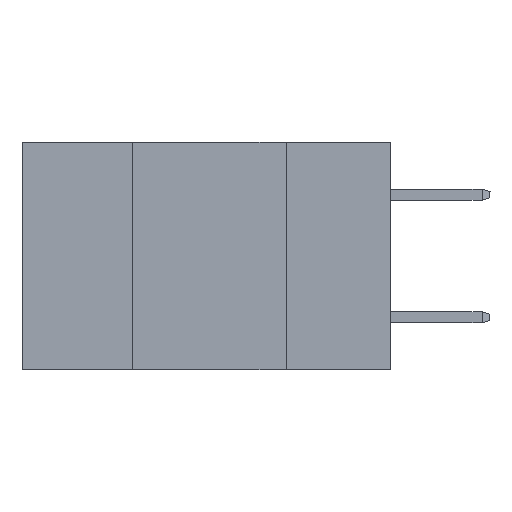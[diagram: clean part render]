
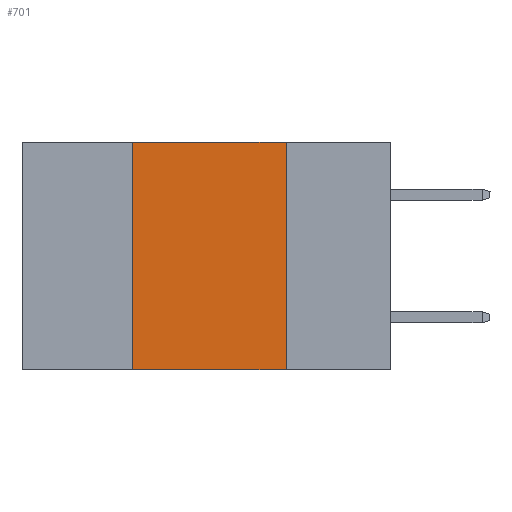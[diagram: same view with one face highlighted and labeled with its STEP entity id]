
A CAD part, left-side view. The second image highlights one B-rep face of the part: STEP entity #701.
In plain terms, the highlighted planar face has unit normal (-1, 0, 0).
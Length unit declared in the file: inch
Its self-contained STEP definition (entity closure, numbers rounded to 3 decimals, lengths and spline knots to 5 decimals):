
#64 = LINE ( 'NONE', #5505, #826 ) ;
#701 = ADVANCED_FACE ( 'NONE', ( #5177 ), #5519, .F. ) ;
#825 = VECTOR ( 'NONE', #9366, 39.37008 ) ;
#826 = VECTOR ( 'NONE', #6324, 39.37008 ) ;
#1001 = LINE ( 'NONE', #8218, #5289 ) ;
#1124 = CARTESIAN_POINT ( 'NONE',  ( 0., 0.6, -0.37 ) ) ;
#1173 = ORIENTED_EDGE ( 'NONE', *, *, #5974, .F. ) ;
#1930 = VERTEX_POINT ( 'NONE', #3570 ) ;
#2139 = CARTESIAN_POINT ( 'NONE',  ( 0., 0.6, 0. ) ) ;
#2370 = CARTESIAN_POINT ( 'NONE',  ( 0., 0.6, 0. ) ) ;
#2545 = EDGE_CURVE ( 'NONE', #3255, #5693, #4524, .T. ) ;
#2856 = EDGE_CURVE ( 'NONE', #4542, #1930, #6290, .T. ) ;
#3011 = DIRECTION ( 'NONE',  ( 0., 0., -1. ) ) ;
#3255 = VERTEX_POINT ( 'NONE', #3882 ) ;
#3570 = CARTESIAN_POINT ( 'NONE',  ( 0., 0.17, 0. ) ) ;
#3882 = CARTESIAN_POINT ( 'NONE',  ( 0., 0.42, -0.37 ) ) ;
#4016 = DIRECTION ( 'NONE',  ( 0., -1., 0. ) ) ;
#4229 = ORIENTED_EDGE ( 'NONE', *, *, #7772, .F. ) ;
#4290 = CARTESIAN_POINT ( 'NONE',  ( 0., 0.17, -0.37 ) ) ;
#4524 = LINE ( 'NONE', #1124, #7410 ) ;
#4542 = VERTEX_POINT ( 'NONE', #6496 ) ;
#5177 = FACE_OUTER_BOUND ( 'NONE', #7313, .T. ) ;
#5289 = VECTOR ( 'NONE', #9020, 39.37008 ) ;
#5505 = CARTESIAN_POINT ( 'NONE',  ( 0., 0.17, 0. ) ) ;
#5519 = PLANE ( 'NONE',  #9348 ) ;
#5693 = VERTEX_POINT ( 'NONE', #4290 ) ;
#5974 = EDGE_CURVE ( 'NONE', #3255, #4542, #1001, .T. ) ;
#6290 = LINE ( 'NONE', #2139, #825 ) ;
#6324 = DIRECTION ( 'NONE',  ( 0., 0., -1. ) ) ;
#6496 = CARTESIAN_POINT ( 'NONE',  ( 0., 0.42, 0. ) ) ;
#7313 = EDGE_LOOP ( 'NONE', ( #4229, #9362, #1173, #8686 ) ) ;
#7410 = VECTOR ( 'NONE', #4016, 39.37008 ) ;
#7772 = EDGE_CURVE ( 'NONE', #1930, #5693, #64, .T. ) ;
#7963 = DIRECTION ( 'NONE',  ( 1., 0., 0. ) ) ;
#8218 = CARTESIAN_POINT ( 'NONE',  ( 0., 0.42, 0. ) ) ;
#8686 = ORIENTED_EDGE ( 'NONE', *, *, #2545, .T. ) ;
#9020 = DIRECTION ( 'NONE',  ( 0., 0., 1. ) ) ;
#9348 = AXIS2_PLACEMENT_3D ( 'NONE', #2370, #7963, #3011 ) ;
#9362 = ORIENTED_EDGE ( 'NONE', *, *, #2856, .F. ) ;
#9366 = DIRECTION ( 'NONE',  ( 0., -1., 0. ) ) ;
